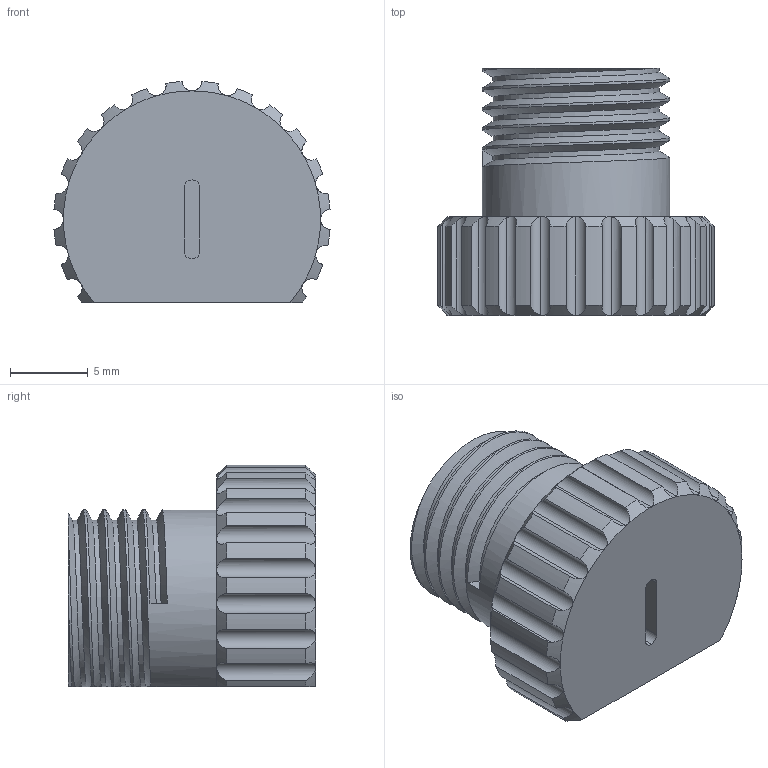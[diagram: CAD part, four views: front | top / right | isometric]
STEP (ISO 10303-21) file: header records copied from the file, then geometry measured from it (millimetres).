
FILE_DESCRIPTION (( 'STEP AP203' ), '1' );
FILE_NAME ('AF-GFP-MP-PRT-003-STEP.STEP', '2020-08-05T21:38:54', ( '' ), ( '' ), 'SwSTEP 2.0', 'SolidWorks 2018', '' );
FILE_SCHEMA (( 'CONFIG_CONTROL_DESIGN' ));
Length unit declared in the file: inch
Products named in the file (1): AF-GFP-MP-PRT-003-STEP
Bounding box: 17.73 x 15.88 x 14.21 mm (x, y, z)
Volume: 2250.9 mm3; surface area: 1284.8 mm2
Topology: 1 solids, 1 shells, 114 faces, 297 edges, 186 vertices
Faces by surface type: cylinder 54, cone 36, bspline 16, plane 8
Entity records: 6830 total; most frequent: CARTESIAN_POINT 4281, ORIENTED_EDGE 594, DIRECTION 429, EDGE_CURVE 297, VERTEX_POINT 186, AXIS2_PLACEMENT_3D 179, B_SPLINE_CURVE_WITH_KNOTS 117, EDGE_LOOP 115
